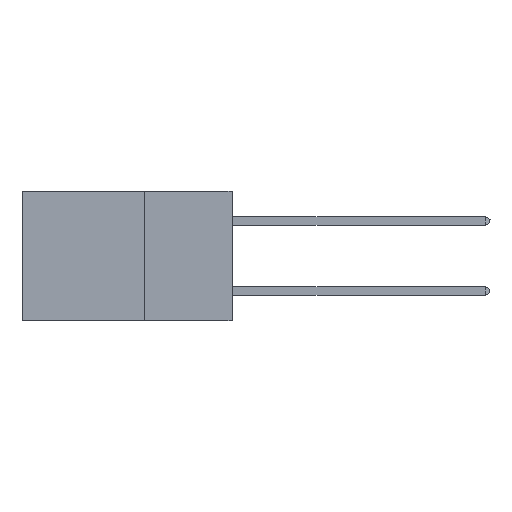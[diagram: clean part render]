
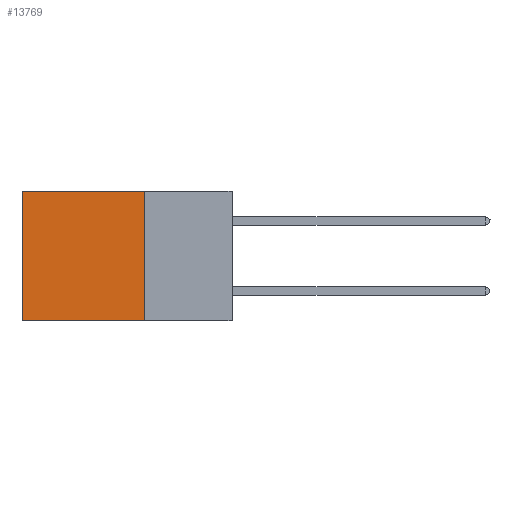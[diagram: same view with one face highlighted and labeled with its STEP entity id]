
A CAD part, left-side view. The second image highlights one B-rep face of the part: STEP entity #13769.
In plain terms, the highlighted planar face has unit normal (-1, 0, 0).
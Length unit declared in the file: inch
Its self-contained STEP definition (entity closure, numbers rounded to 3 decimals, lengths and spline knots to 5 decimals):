
#464 = DIRECTION ( 'NONE',  ( 0., 1., 0. ) ) ;
#492 = EDGE_CURVE ( 'NONE', #7659, #15743, #18869, .T. ) ;
#676 = EDGE_CURVE ( 'NONE', #18728, #7659, #7937, .T. ) ;
#1964 = CARTESIAN_POINT ( 'NONE',  ( 0.2875, 0.6, 0. ) ) ;
#2561 = VERTEX_POINT ( 'NONE', #5932 ) ;
#2914 = CARTESIAN_POINT ( 'NONE',  ( 0.2875, 0.6, -0.37 ) ) ;
#3238 = ORIENTED_EDGE ( 'NONE', *, *, #4326, .F. ) ;
#3254 = CARTESIAN_POINT ( 'NONE',  ( 0.2875, 0.25, 0. ) ) ;
#3520 = DIRECTION ( 'NONE',  ( 0., 0., -1. ) ) ;
#3873 = VECTOR ( 'NONE', #15104, 39.37008 ) ;
#4326 = EDGE_CURVE ( 'NONE', #2561, #15743, #4679, .T. ) ;
#4564 = EDGE_CURVE ( 'NONE', #18728, #2561, #13620, .T. ) ;
#4679 = LINE ( 'NONE', #18694, #10470 ) ;
#5932 = CARTESIAN_POINT ( 'NONE',  ( 0.2875, 0.25, -0.37 ) ) ;
#5934 = ORIENTED_EDGE ( 'NONE', *, *, #4564, .F. ) ;
#6511 = VECTOR ( 'NONE', #3520, 39.37008 ) ;
#7594 = DIRECTION ( 'NONE',  ( 0., 0., -1. ) ) ;
#7659 = VERTEX_POINT ( 'NONE', #7774 ) ;
#7701 = FACE_OUTER_BOUND ( 'NONE', #16814, .T. ) ;
#7774 = CARTESIAN_POINT ( 'NONE',  ( 0.2875, 0.6, 0. ) ) ;
#7875 = DIRECTION ( 'NONE',  ( 0., 0., -1. ) ) ;
#7937 = LINE ( 'NONE', #11928, #3873 ) ;
#9934 = ORIENTED_EDGE ( 'NONE', *, *, #676, .T. ) ;
#10470 = VECTOR ( 'NONE', #464, 39.37008 ) ;
#11928 = CARTESIAN_POINT ( 'NONE',  ( 0.2875, 0.25, 0. ) ) ;
#12172 = AXIS2_PLACEMENT_3D ( 'NONE', #14097, #15461, #7594 ) ;
#12400 = VECTOR ( 'NONE', #7875, 39.37008 ) ;
#12480 = PLANE ( 'NONE',  #12172 ) ;
#13620 = LINE ( 'NONE', #3254, #12400 ) ;
#13769 = ADVANCED_FACE ( 'NONE', ( #7701 ), #12480, .F. ) ;
#14097 = CARTESIAN_POINT ( 'NONE',  ( 0.2875, 0.25, 0. ) ) ;
#15104 = DIRECTION ( 'NONE',  ( 0., 1., 0. ) ) ;
#15461 = DIRECTION ( 'NONE',  ( 1., 0., 0. ) ) ;
#15743 = VERTEX_POINT ( 'NONE', #2914 ) ;
#16321 = CARTESIAN_POINT ( 'NONE',  ( 0.2875, 0.25, 0. ) ) ;
#16814 = EDGE_LOOP ( 'NONE', ( #17518, #3238, #5934, #9934 ) ) ;
#17518 = ORIENTED_EDGE ( 'NONE', *, *, #492, .T. ) ;
#18694 = CARTESIAN_POINT ( 'NONE',  ( 0.2875, 0.25, -0.37 ) ) ;
#18728 = VERTEX_POINT ( 'NONE', #16321 ) ;
#18869 = LINE ( 'NONE', #1964, #6511 ) ;
